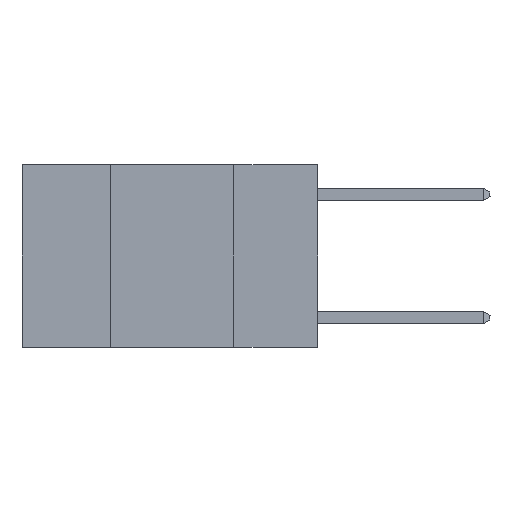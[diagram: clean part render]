
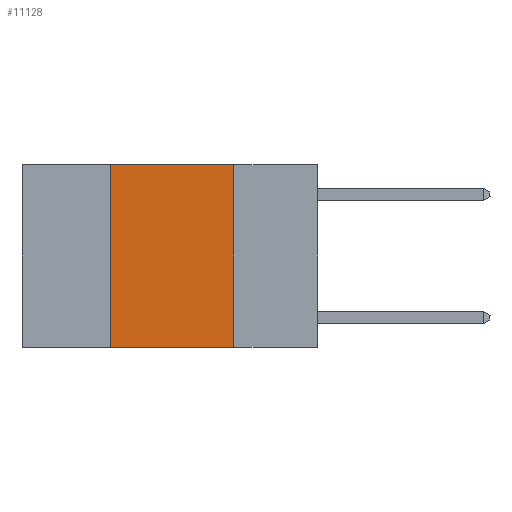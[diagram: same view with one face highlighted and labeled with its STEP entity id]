
A CAD part, left-side view. The second image highlights one B-rep face of the part: STEP entity #11128.
In plain terms, the highlighted planar face has unit normal (-1, 0, 0).
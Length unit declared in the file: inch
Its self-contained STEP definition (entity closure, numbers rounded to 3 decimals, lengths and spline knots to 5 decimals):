
#5 = EDGE_CURVE ( 'NONE', #4210, #12338, #11092, .T. ) ;
#427 = CARTESIAN_POINT ( 'NONE',  ( 0., 0.6, 0. ) ) ;
#843 = ORIENTED_EDGE ( 'NONE', *, *, #9403, .F. ) ;
#1112 = CARTESIAN_POINT ( 'NONE',  ( 0., 0.6, 0. ) ) ;
#1829 = ORIENTED_EDGE ( 'NONE', *, *, #12874, .T. ) ;
#1848 = DIRECTION ( 'NONE',  ( 0., -1., 0. ) ) ;
#1906 = CARTESIAN_POINT ( 'NONE',  ( 0., 0.42, 0. ) ) ;
#2160 = LINE ( 'NONE', #4963, #6963 ) ;
#2175 = DIRECTION ( 'NONE',  ( 0., 0., -1. ) ) ;
#3299 = ORIENTED_EDGE ( 'NONE', *, *, #6892, .F. ) ;
#3693 = VERTEX_POINT ( 'NONE', #9772 ) ;
#4210 = VERTEX_POINT ( 'NONE', #8791 ) ;
#4963 = CARTESIAN_POINT ( 'NONE',  ( 0., 0.6, -0.37 ) ) ;
#5092 = FACE_OUTER_BOUND ( 'NONE', #6225, .T. ) ;
#5540 = AXIS2_PLACEMENT_3D ( 'NONE', #1112, #8240, #2175 ) ;
#5836 = DIRECTION ( 'NONE',  ( 0., 0., 1. ) ) ;
#6225 = EDGE_LOOP ( 'NONE', ( #3299, #843, #11961, #1829 ) ) ;
#6774 = CARTESIAN_POINT ( 'NONE',  ( 0., 0.42, 0. ) ) ;
#6892 = EDGE_CURVE ( 'NONE', #9064, #3693, #9045, .T. ) ;
#6963 = VECTOR ( 'NONE', #1848, 39.37008 ) ;
#7257 = PLANE ( 'NONE',  #5540 ) ;
#8240 = DIRECTION ( 'NONE',  ( 1., 0., 0. ) ) ;
#8406 = VECTOR ( 'NONE', #5836, 39.37008 ) ;
#8775 = DIRECTION ( 'NONE',  ( 0., 0., -1. ) ) ;
#8791 = CARTESIAN_POINT ( 'NONE',  ( 0., 0.42, -0.37 ) ) ;
#9045 = LINE ( 'NONE', #10772, #11742 ) ;
#9064 = VERTEX_POINT ( 'NONE', #12105 ) ;
#9403 = EDGE_CURVE ( 'NONE', #12338, #9064, #12119, .T. ) ;
#9759 = VECTOR ( 'NONE', #11592, 39.37008 ) ;
#9772 = CARTESIAN_POINT ( 'NONE',  ( 0., 0.17, -0.37 ) ) ;
#10772 = CARTESIAN_POINT ( 'NONE',  ( 0., 0.17, 0. ) ) ;
#11092 = LINE ( 'NONE', #6774, #8406 ) ;
#11128 = ADVANCED_FACE ( 'NONE', ( #5092 ), #7257, .F. ) ;
#11592 = DIRECTION ( 'NONE',  ( 0., -1., 0. ) ) ;
#11742 = VECTOR ( 'NONE', #8775, 39.37008 ) ;
#11961 = ORIENTED_EDGE ( 'NONE', *, *, #5, .F. ) ;
#12105 = CARTESIAN_POINT ( 'NONE',  ( 0., 0.17, 0. ) ) ;
#12119 = LINE ( 'NONE', #427, #9759 ) ;
#12338 = VERTEX_POINT ( 'NONE', #1906 ) ;
#12874 = EDGE_CURVE ( 'NONE', #4210, #3693, #2160, .T. ) ;
